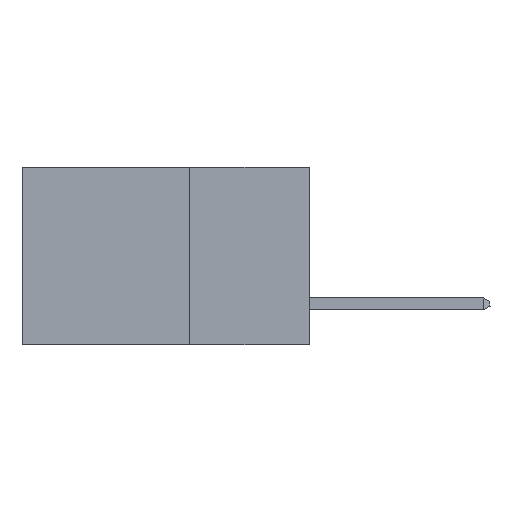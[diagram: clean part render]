
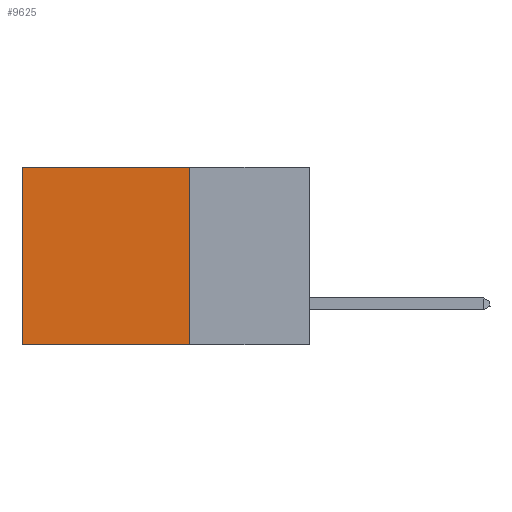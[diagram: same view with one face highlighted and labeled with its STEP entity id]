
A CAD part, left-side view. The second image highlights one B-rep face of the part: STEP entity #9625.
In plain terms, the highlighted planar face has unit normal (-1, 0, 0).
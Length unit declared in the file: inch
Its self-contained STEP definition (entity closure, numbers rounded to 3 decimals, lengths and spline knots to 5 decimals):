
#614 = EDGE_LOOP ( 'NONE', ( #6767, #19240, #11577, #7887 ) ) ;
#1282 = VECTOR ( 'NONE', #11249, 39.37008 ) ;
#1761 = CARTESIAN_POINT ( 'NONE',  ( 0.2875, 0.25, 0. ) ) ;
#1909 = VECTOR ( 'NONE', #8392, 39.37008 ) ;
#2753 = EDGE_CURVE ( 'NONE', #19578, #16603, #5343, .T. ) ;
#3037 = AXIS2_PLACEMENT_3D ( 'NONE', #12854, #8255, #12924 ) ;
#3958 = DIRECTION ( 'NONE',  ( 0., 1., 0. ) ) ;
#4126 = LINE ( 'NONE', #13064, #10436 ) ;
#4274 = EDGE_CURVE ( 'NONE', #16603, #5703, #4126, .T. ) ;
#4781 = LINE ( 'NONE', #13138, #1909 ) ;
#5343 = LINE ( 'NONE', #1761, #1282 ) ;
#5703 = VERTEX_POINT ( 'NONE', #6093 ) ;
#6093 = CARTESIAN_POINT ( 'NONE',  ( 0.2875, 0.6, -0.37 ) ) ;
#6767 = ORIENTED_EDGE ( 'NONE', *, *, #12781, .T. ) ;
#7887 = ORIENTED_EDGE ( 'NONE', *, *, #19470, .T. ) ;
#8255 = DIRECTION ( 'NONE',  ( 1., 0., 0. ) ) ;
#8392 = DIRECTION ( 'NONE',  ( 0., 1., 0. ) ) ;
#9625 = ADVANCED_FACE ( 'NONE', ( #14544 ), #14685, .F. ) ;
#9766 = DIRECTION ( 'NONE',  ( 0., 0., -1. ) ) ;
#10396 = CARTESIAN_POINT ( 'NONE',  ( 0.2875, 0.25, 0. ) ) ;
#10436 = VECTOR ( 'NONE', #3958, 39.37008 ) ;
#10786 = VERTEX_POINT ( 'NONE', #16762 ) ;
#10840 = CARTESIAN_POINT ( 'NONE',  ( 0.2875, 0.25, -0.37 ) ) ;
#11249 = DIRECTION ( 'NONE',  ( 0., 0., -1. ) ) ;
#11577 = ORIENTED_EDGE ( 'NONE', *, *, #2753, .F. ) ;
#11781 = LINE ( 'NONE', #15880, #12460 ) ;
#12460 = VECTOR ( 'NONE', #9766, 39.37008 ) ;
#12781 = EDGE_CURVE ( 'NONE', #10786, #5703, #11781, .T. ) ;
#12854 = CARTESIAN_POINT ( 'NONE',  ( 0.2875, 0.25, 0. ) ) ;
#12924 = DIRECTION ( 'NONE',  ( 0., 0., -1. ) ) ;
#13064 = CARTESIAN_POINT ( 'NONE',  ( 0.2875, 0.25, -0.37 ) ) ;
#13138 = CARTESIAN_POINT ( 'NONE',  ( 0.2875, 0.25, 0. ) ) ;
#14544 = FACE_OUTER_BOUND ( 'NONE', #614, .T. ) ;
#14685 = PLANE ( 'NONE',  #3037 ) ;
#15880 = CARTESIAN_POINT ( 'NONE',  ( 0.2875, 0.6, 0. ) ) ;
#16603 = VERTEX_POINT ( 'NONE', #10840 ) ;
#16762 = CARTESIAN_POINT ( 'NONE',  ( 0.2875, 0.6, 0. ) ) ;
#19240 = ORIENTED_EDGE ( 'NONE', *, *, #4274, .F. ) ;
#19470 = EDGE_CURVE ( 'NONE', #19578, #10786, #4781, .T. ) ;
#19578 = VERTEX_POINT ( 'NONE', #10396 ) ;
